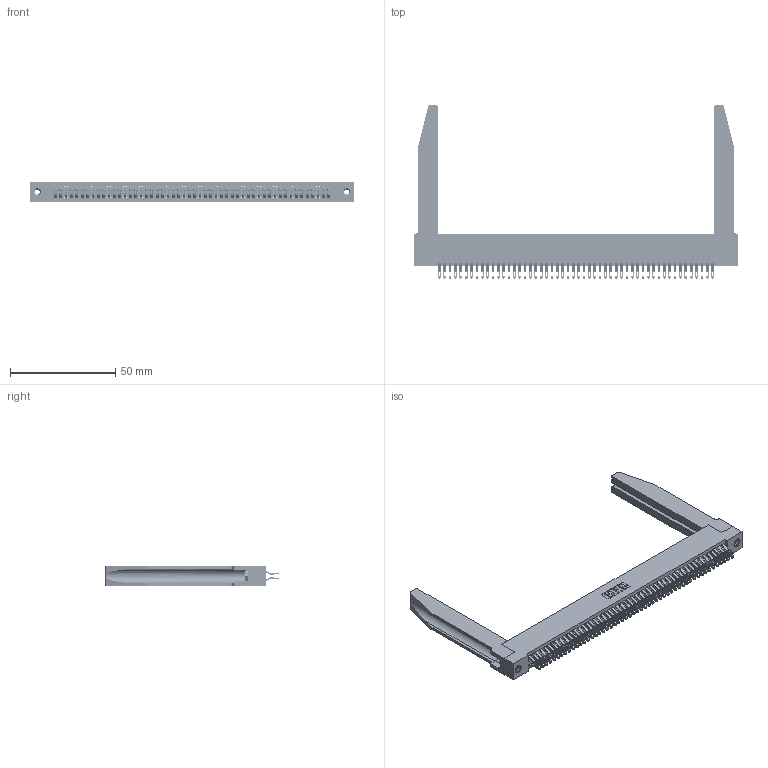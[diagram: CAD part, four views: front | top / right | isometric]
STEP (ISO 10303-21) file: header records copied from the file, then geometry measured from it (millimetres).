
FILE_DESCRIPTION (( 'STEP AP203' ), '1' );
FILE_NAME ('345-104-555-278.STEP', '2019-11-03T12:34:20', ( '' ), ( '' ), 'SwSTEP 2.0', 'SolidWorks 2016', '' );
FILE_SCHEMA (( 'CONFIG_CONTROL_DESIGN' ));
Length unit declared in the file: inch
Products named in the file (5): 345-250-001_345-250-001-102; 345 Part_Flush Mounting Lugs - 0.156 Dia-TH; 345-292-001_555 Tail; 345-104-555-278; 345-220-078_345-220-078
Assembly tree (109 placements, depth 2):
  345-104-555-278
    345 Part_Flush Mounting Lugs - 0.156 Dia-TH
    345-292-001_555 Tail  x104
    345-250-001_345-250-001-102  x2
    345-220-078_345-220-078  x2
Bounding box: 153.31 x 82.09 x 9.4 mm (x, y, z)
Volume: 23058 mm3; surface area: 30679 mm2
Topology: 109 solids, 109 shells, 6184 faces, 19357 edges, 12894 vertices
Faces by surface type: plane 3446, cylinder 2686, bspline 36, cone 12, torus 4
Entity records: 44520 total; most frequent: CARTESIAN_POINT 8405, ORIENTED_EDGE 7206, DIRECTION 6361, EDGE_CURVE 3603, VECTOR 3149, LINE 3149, VERTEX_POINT 2396, AXIS2_PLACEMENT_3D 1606
